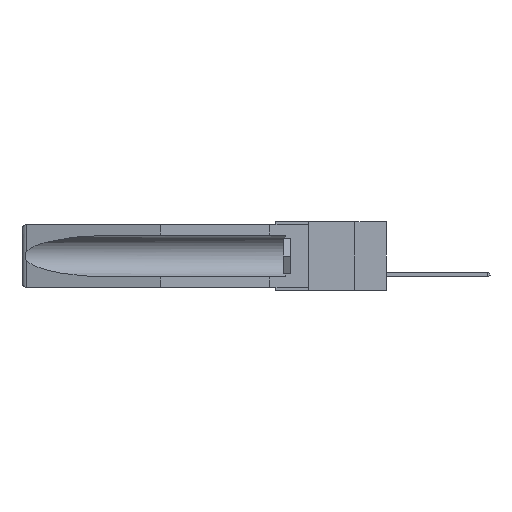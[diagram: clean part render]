
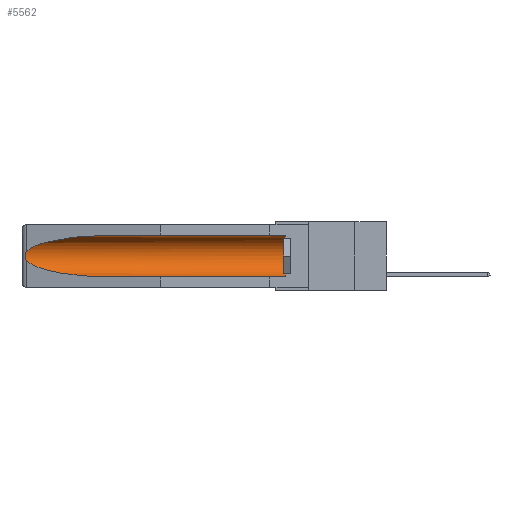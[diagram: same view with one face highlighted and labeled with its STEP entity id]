
A CAD part, left-side view. The second image highlights one B-rep face of the part: STEP entity #5562.
In plain terms, the highlighted cylindrical face has radius 2.857 mm (diameter 5.715 mm), a partial arc.
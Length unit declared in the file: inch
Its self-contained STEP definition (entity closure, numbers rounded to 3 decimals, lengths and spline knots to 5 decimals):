
#532 = VERTEX_POINT ( 'NONE', #3694 ) ;
#783 = VERTEX_POINT ( 'NONE', #18729 ) ;
#938 = CARTESIAN_POINT ( 'NONE',  ( 0.2673, 1.5327, -0.16383 ) ) ;
#1012 = CARTESIAN_POINT ( 'NONE',  ( 0.26655, 1.53094, -0.18657 ) ) ;
#1115 = CARTESIAN_POINT ( 'NONE',  ( 0.21114, 1.30732, -0.059 ) ) ;
#2155 = EDGE_LOOP ( 'NONE', ( #8737, #16893, #11679, #14962, #18913, #7785 ) ) ;
#2435 = CARTESIAN_POINT ( 'NONE',  ( 0.155, 0.126, -0.284 ) ) ;
#2824 = CARTESIAN_POINT ( 'NONE',  ( 0.26537, 1.52718, -0.14972 ) ) ;
#3372 = EDGE_CURVE ( 'NONE', #12632, #13419, #3555, .T. ) ;
#3555 = CIRCLE ( 'NONE', #10415, 0.1125 ) ;
#3600 = DIRECTION ( 'NONE',  ( 0., -1., 0. ) ) ;
#3694 = CARTESIAN_POINT ( 'NONE',  ( 0.26537, 1.52718, -0.19328 ) ) ;
#4033 =( BOUNDED_CURVE ( )  B_SPLINE_CURVE ( 3, ( #6374, #1115, #15613, #2824 ),
 .UNSPECIFIED., .F., .F. ) 
 B_SPLINE_CURVE_WITH_KNOTS ( ( 4, 4 ),
 ( 4.71239, 6.08839 ),
 .UNSPECIFIED. ) 
 CURVE ( )  GEOMETRIC_REPRESENTATION_ITEM ( )  RATIONAL_B_SPLINE_CURVE ( ( 1., 0.848, 0.848, 1. ) ) 
 REPRESENTATION_ITEM ( '' )  );
#4540 = CARTESIAN_POINT ( 'NONE',  ( 0.26537, 1.52718, -0.19328 ) ) ;
#5562 = ADVANCED_FACE ( 'NONE', ( #18211 ), #11965, .F. ) ;
#6285 = VECTOR ( 'NONE', #10633, 39.37008 ) ;
#6374 = CARTESIAN_POINT ( 'NONE',  ( 0.155, 1.07973, -0.059 ) ) ;
#6524 = B_SPLINE_CURVE_WITH_KNOTS ( 'NONE', 3,
 ( #22642, #13597, #15273, #938, #22418, #11830, #8039, #1012, #20798, #4540 ),
 .UNSPECIFIED., .F., .F.,
 ( 4, 2, 2, 2, 4 ),
 ( 0., 0.00029, 0.00058, 0.00087, 0.00117 ),
 .UNSPECIFIED. ) ;
#6724 = DIRECTION ( 'NONE',  ( 0., 1., 0. ) ) ;
#6768 = VECTOR ( 'NONE', #6724, 39.37008 ) ;
#6856 = CARTESIAN_POINT ( 'NONE',  ( 0.155, -0.30754, -0.1715 ) ) ;
#6955 = CARTESIAN_POINT ( 'NONE',  ( 0.155, -0.30754, -0.059 ) ) ;
#7164 = EDGE_CURVE ( 'NONE', #22312, #22806, #4033, .T. ) ;
#7785 = ORIENTED_EDGE ( 'NONE', *, *, #18227, .T. ) ;
#8021 = AXIS2_PLACEMENT_3D ( 'NONE', #6856, #13943, #23048 ) ;
#8039 = CARTESIAN_POINT ( 'NONE',  ( 0.2673, 1.53269, -0.17917 ) ) ;
#8737 = ORIENTED_EDGE ( 'NONE', *, *, #7164, .T. ) ;
#9050 = LINE ( 'NONE', #6955, #6768 ) ;
#9593 = EDGE_CURVE ( 'NONE', #12632, #783, #11948, .T. ) ;
#10415 = AXIS2_PLACEMENT_3D ( 'NONE', #21661, #3600, #10898 ) ;
#10467 = CARTESIAN_POINT ( 'NONE',  ( 0.155, 0.126, -0.059 ) ) ;
#10633 = DIRECTION ( 'NONE',  ( 0., 1., 0. ) ) ;
#10898 = DIRECTION ( 'NONE',  ( 0., 0., 1. ) ) ;
#11679 = ORIENTED_EDGE ( 'NONE', *, *, #12046, .T. ) ;
#11830 = CARTESIAN_POINT ( 'NONE',  ( 0.2675, 1.53308, -0.17534 ) ) ;
#11948 = LINE ( 'NONE', #19685, #6285 ) ;
#11965 = CYLINDRICAL_SURFACE ( 'NONE', #8021, 0.1125 ) ;
#12046 = EDGE_CURVE ( 'NONE', #532, #783, #19182, .T. ) ;
#12632 = VERTEX_POINT ( 'NONE', #2435 ) ;
#13419 = VERTEX_POINT ( 'NONE', #10467 ) ;
#13597 = CARTESIAN_POINT ( 'NONE',  ( 0.26597, 1.52961, -0.15275 ) ) ;
#13748 = CARTESIAN_POINT ( 'NONE',  ( 0.26537, 1.52718, -0.14972 ) ) ;
#13943 = DIRECTION ( 'NONE',  ( 0., 1., 0. ) ) ;
#14470 = CARTESIAN_POINT ( 'NONE',  ( 0.155, 1.07973, -0.284 ) ) ;
#14962 = ORIENTED_EDGE ( 'NONE', *, *, #9593, .F. ) ;
#15273 = CARTESIAN_POINT ( 'NONE',  ( 0.26654, 1.53092, -0.15636 ) ) ;
#15613 = CARTESIAN_POINT ( 'NONE',  ( 0.25451, 1.48313, -0.09465 ) ) ;
#16212 = CARTESIAN_POINT ( 'NONE',  ( 0.21114, 1.30732, -0.284 ) ) ;
#16289 = CARTESIAN_POINT ( 'NONE',  ( 0.26537, 1.52718, -0.19328 ) ) ;
#16893 = ORIENTED_EDGE ( 'NONE', *, *, #22774, .T. ) ;
#17975 = CARTESIAN_POINT ( 'NONE',  ( 0.155, 1.07973, -0.059 ) ) ;
#18211 = FACE_OUTER_BOUND ( 'NONE', #2155, .T. ) ;
#18227 = EDGE_CURVE ( 'NONE', #13419, #22312, #9050, .T. ) ;
#18729 = CARTESIAN_POINT ( 'NONE',  ( 0.155, 1.07973, -0.284 ) ) ;
#18913 = ORIENTED_EDGE ( 'NONE', *, *, #3372, .T. ) ;
#19182 =( BOUNDED_CURVE ( )  B_SPLINE_CURVE ( 3, ( #16289, #21714, #16212, #14470 ),
 .UNSPECIFIED., .F., .F. ) 
 B_SPLINE_CURVE_WITH_KNOTS ( ( 4, 4 ),
 ( 0.1948, 1.5708 ),
 .UNSPECIFIED. ) 
 CURVE ( )  GEOMETRIC_REPRESENTATION_ITEM ( )  RATIONAL_B_SPLINE_CURVE ( ( 1., 0.848, 0.848, 1. ) ) 
 REPRESENTATION_ITEM ( '' )  );
#19685 = CARTESIAN_POINT ( 'NONE',  ( 0.155, -0.30754, -0.284 ) ) ;
#20798 = CARTESIAN_POINT ( 'NONE',  ( 0.26597, 1.5296, -0.19026 ) ) ;
#21661 = CARTESIAN_POINT ( 'NONE',  ( 0.155, 0.126, -0.1715 ) ) ;
#21714 = CARTESIAN_POINT ( 'NONE',  ( 0.25451, 1.48313, -0.24835 ) ) ;
#22312 = VERTEX_POINT ( 'NONE', #17975 ) ;
#22418 = CARTESIAN_POINT ( 'NONE',  ( 0.2675, 1.53308, -0.16763 ) ) ;
#22642 = CARTESIAN_POINT ( 'NONE',  ( 0.26537, 1.52718, -0.14972 ) ) ;
#22774 = EDGE_CURVE ( 'NONE', #22806, #532, #6524, .T. ) ;
#22806 = VERTEX_POINT ( 'NONE', #13748 ) ;
#23048 = DIRECTION ( 'NONE',  ( 0., 0., 1. ) ) ;
